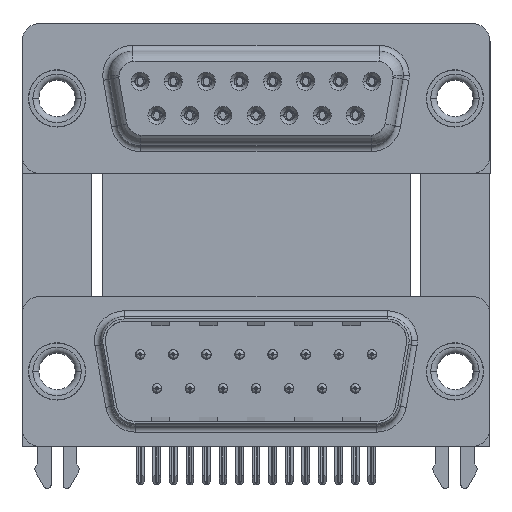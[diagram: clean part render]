
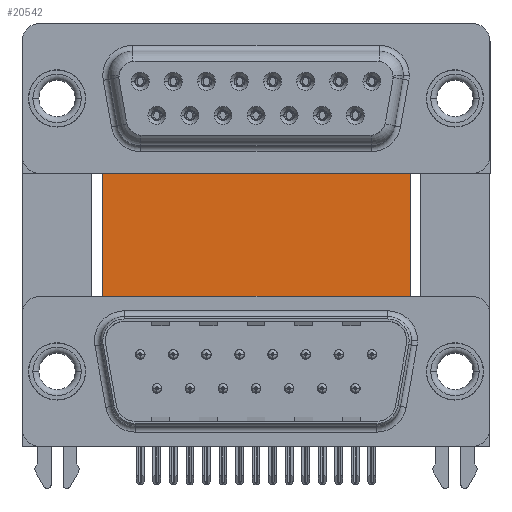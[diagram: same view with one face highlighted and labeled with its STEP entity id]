
A CAD part, top view. The second image highlights one B-rep face of the part: STEP entity #20542.
In plain terms, the highlighted planar face has unit normal (0, 0, 1).
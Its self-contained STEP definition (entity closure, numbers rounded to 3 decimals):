
#1154 = AXIS2_PLACEMENT_3D ( 'NONE', #35559, #35766, #38643 ) ;
#1512 = LINE ( 'NONE', #8733, #8904 ) ;
#3577 = VERTEX_POINT ( 'NONE', #25516 ) ;
#5523 = VERTEX_POINT ( 'NONE', #15409 ) ;
#6283 = CARTESIAN_POINT ( 'NONE',  ( 3.79, -3.735, -12. ) ) ;
#6582 = ORIENTED_EDGE ( 'NONE', *, *, #33505, .F. ) ;
#7996 = VECTOR ( 'NONE', #21100, 1000. ) ;
#8550 = VECTOR ( 'NONE', #22444, 1000. ) ;
#8733 = CARTESIAN_POINT ( 'NONE',  ( 3.79, 16.585, -12. ) ) ;
#8904 = VECTOR ( 'NONE', #11610, 1000. ) ;
#9029 = CARTESIAN_POINT ( 'NONE',  ( 3.79, 16.585, -12. ) ) ;
#10994 = LINE ( 'NONE', #13869, #7996 ) ;
#11610 = DIRECTION ( 'NONE',  ( 0., -1., 0. ) ) ;
#12518 = ORIENTED_EDGE ( 'NONE', *, *, #29878, .F. ) ;
#13137 = EDGE_CURVE ( 'NONE', #3577, #15373, #1512, .T. ) ;
#13869 = CARTESIAN_POINT ( 'NONE',  ( 29.58, 16.585, -12. ) ) ;
#14042 = CARTESIAN_POINT ( 'NONE',  ( 3.79, -3.735, -12. ) ) ;
#15373 = VERTEX_POINT ( 'NONE', #14042 ) ;
#15409 = CARTESIAN_POINT ( 'NONE',  ( 29.58, 16.585, -12. ) ) ;
#18177 = FACE_OUTER_BOUND ( 'NONE', #33215, .T. ) ;
#19037 = VECTOR ( 'NONE', #26727, 1000. ) ;
#20542 = ADVANCED_FACE ( 'NONE', ( #18177 ), #41962, .F. ) ;
#21100 = DIRECTION ( 'NONE',  ( 0., -1., 0. ) ) ;
#22444 = DIRECTION ( 'NONE',  ( 1., 0., 0. ) ) ;
#25071 = VERTEX_POINT ( 'NONE', #37675 ) ;
#25516 = CARTESIAN_POINT ( 'NONE',  ( 3.79, 16.585, -12. ) ) ;
#26078 = LINE ( 'NONE', #6283, #19037 ) ;
#26727 = DIRECTION ( 'NONE',  ( 1., 0., 0. ) ) ;
#27054 = EDGE_CURVE ( 'NONE', #15373, #25071, #26078, .T. ) ;
#29878 = EDGE_CURVE ( 'NONE', #3577, #5523, #39178, .T. ) ;
#31684 = ORIENTED_EDGE ( 'NONE', *, *, #27054, .T. ) ;
#33215 = EDGE_LOOP ( 'NONE', ( #31684, #6582, #12518, #42457 ) ) ;
#33505 = EDGE_CURVE ( 'NONE', #5523, #25071, #10994, .T. ) ;
#35559 = CARTESIAN_POINT ( 'NONE',  ( 3.79, 16.585, -12. ) ) ;
#35766 = DIRECTION ( 'NONE',  ( 0., 0., -1. ) ) ;
#37675 = CARTESIAN_POINT ( 'NONE',  ( 29.58, -3.735, -12. ) ) ;
#38643 = DIRECTION ( 'NONE',  ( -1., 0., 0. ) ) ;
#39178 = LINE ( 'NONE', #9029, #8550 ) ;
#41962 = PLANE ( 'NONE',  #1154 ) ;
#42457 = ORIENTED_EDGE ( 'NONE', *, *, #13137, .T. ) ;
